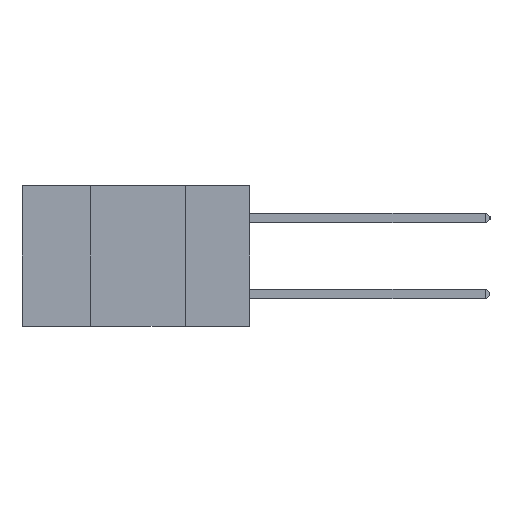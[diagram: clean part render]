
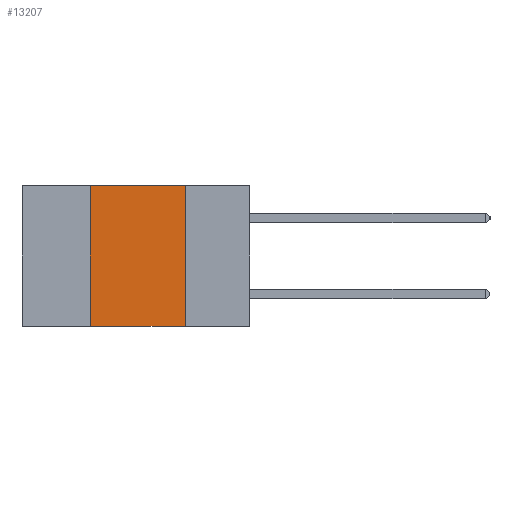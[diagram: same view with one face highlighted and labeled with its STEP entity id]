
A CAD part, left-side view. The second image highlights one B-rep face of the part: STEP entity #13207.
In plain terms, the highlighted planar face has unit normal (-1, 0, 0).
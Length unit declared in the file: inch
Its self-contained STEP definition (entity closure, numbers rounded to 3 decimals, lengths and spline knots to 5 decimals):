
#214 = DIRECTION ( 'NONE',  ( 0., -1., 0. ) ) ;
#768 = VERTEX_POINT ( 'NONE', #7386 ) ;
#962 = ORIENTED_EDGE ( 'NONE', *, *, #9239, .F. ) ;
#1120 = DIRECTION ( 'NONE',  ( 0., 0., -1. ) ) ;
#1250 = LINE ( 'NONE', #13853, #9839 ) ;
#1352 = EDGE_CURVE ( 'NONE', #768, #12237, #7350, .T. ) ;
#1753 = EDGE_CURVE ( 'NONE', #3152, #2512, #1250, .T. ) ;
#2272 = VECTOR ( 'NONE', #11423, 39.37008 ) ;
#2512 = VERTEX_POINT ( 'NONE', #5110 ) ;
#3152 = VERTEX_POINT ( 'NONE', #11868 ) ;
#4102 = LINE ( 'NONE', #10400, #9611 ) ;
#4613 = EDGE_LOOP ( 'NONE', ( #9028, #6262, #962, #9818 ) ) ;
#4678 = FACE_OUTER_BOUND ( 'NONE', #4613, .T. ) ;
#4791 = AXIS2_PLACEMENT_3D ( 'NONE', #11126, #7973, #1120 ) ;
#5110 = CARTESIAN_POINT ( 'NONE',  ( 0., 0.17, -0.37 ) ) ;
#6262 = ORIENTED_EDGE ( 'NONE', *, *, #1352, .F. ) ;
#7178 = CARTESIAN_POINT ( 'NONE',  ( 0., 0.42, 0. ) ) ;
#7350 = LINE ( 'NONE', #13807, #10510 ) ;
#7386 = CARTESIAN_POINT ( 'NONE',  ( 0., 0.42, 0. ) ) ;
#7767 = DIRECTION ( 'NONE',  ( 0., -1., 0. ) ) ;
#7973 = DIRECTION ( 'NONE',  ( 1., 0., 0. ) ) ;
#8237 = LINE ( 'NONE', #7178, #2272 ) ;
#9028 = ORIENTED_EDGE ( 'NONE', *, *, #13449, .F. ) ;
#9239 = EDGE_CURVE ( 'NONE', #3152, #768, #8237, .T. ) ;
#9611 = VECTOR ( 'NONE', #11484, 39.37008 ) ;
#9818 = ORIENTED_EDGE ( 'NONE', *, *, #1753, .T. ) ;
#9839 = VECTOR ( 'NONE', #7767, 39.37008 ) ;
#10400 = CARTESIAN_POINT ( 'NONE',  ( 0., 0.17, 0. ) ) ;
#10510 = VECTOR ( 'NONE', #214, 39.37008 ) ;
#11126 = CARTESIAN_POINT ( 'NONE',  ( 0., 0.6, 0. ) ) ;
#11423 = DIRECTION ( 'NONE',  ( 0., 0., 1. ) ) ;
#11484 = DIRECTION ( 'NONE',  ( 0., 0., -1. ) ) ;
#11868 = CARTESIAN_POINT ( 'NONE',  ( 0., 0.42, -0.37 ) ) ;
#12237 = VERTEX_POINT ( 'NONE', #12975 ) ;
#12975 = CARTESIAN_POINT ( 'NONE',  ( 0., 0.17, 0. ) ) ;
#13207 = ADVANCED_FACE ( 'NONE', ( #4678 ), #14198, .F. ) ;
#13449 = EDGE_CURVE ( 'NONE', #12237, #2512, #4102, .T. ) ;
#13807 = CARTESIAN_POINT ( 'NONE',  ( 0., 0.6, 0. ) ) ;
#13853 = CARTESIAN_POINT ( 'NONE',  ( 0., 0.6, -0.37 ) ) ;
#14198 = PLANE ( 'NONE',  #4791 ) ;
